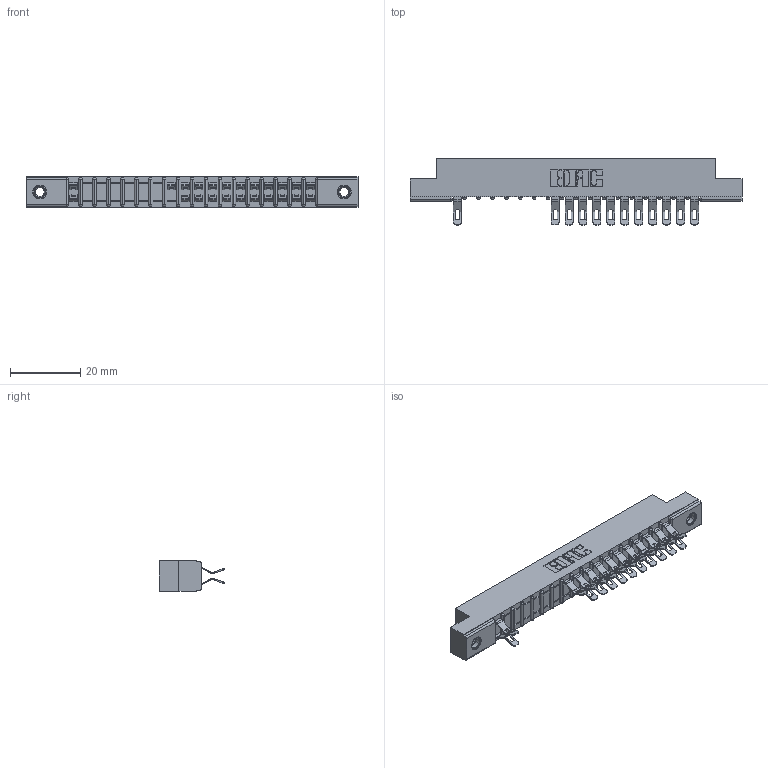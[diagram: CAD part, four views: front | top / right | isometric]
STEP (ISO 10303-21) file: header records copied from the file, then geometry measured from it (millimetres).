
FILE_DESCRIPTION (( 'STEP AP203' ), '1' );
FILE_NAME ('307-036-555-207.STEP', '2018-08-05T09:07:09', ( '' ), ( '' ), 'SwSTEP 2.0', 'SolidWorks 2016', '' );
FILE_SCHEMA (( 'CONFIG_CONTROL_DESIGN' ));
Length unit declared in the file: inch
Products named in the file (4): 307-036-555-207; 307 Part_.156 Dia Mounting Holes; 307-290-001_555; 345-250-001_345-250-005-103
Assembly tree (26 placements, depth 2):
  307-036-555-207
    307 Part_.156 Dia Mounting Holes
    307-290-001_555  x23
    345-250-001_345-250-005-103  x2
Bounding box: 94.34 x 18.75 x 8.71 mm (x, y, z)
Volume: 6057.7 mm3; surface area: 9913.4 mm2
Topology: 26 solids, 26 shells, 1730 faces, 5038 edges, 3268 vertices
Faces by surface type: plane 962, cylinder 714, sphere 38, cone 12, torus 4
Entity records: 20272 total; most frequent: CARTESIAN_POINT 3368, ORIENTED_EDGE 3344, DIRECTION 3312, EDGE_CURVE 1672, VECTOR 1260, LINE 1260, VERTEX_POINT 1082, AXIS2_PLACEMENT_3D 1026
